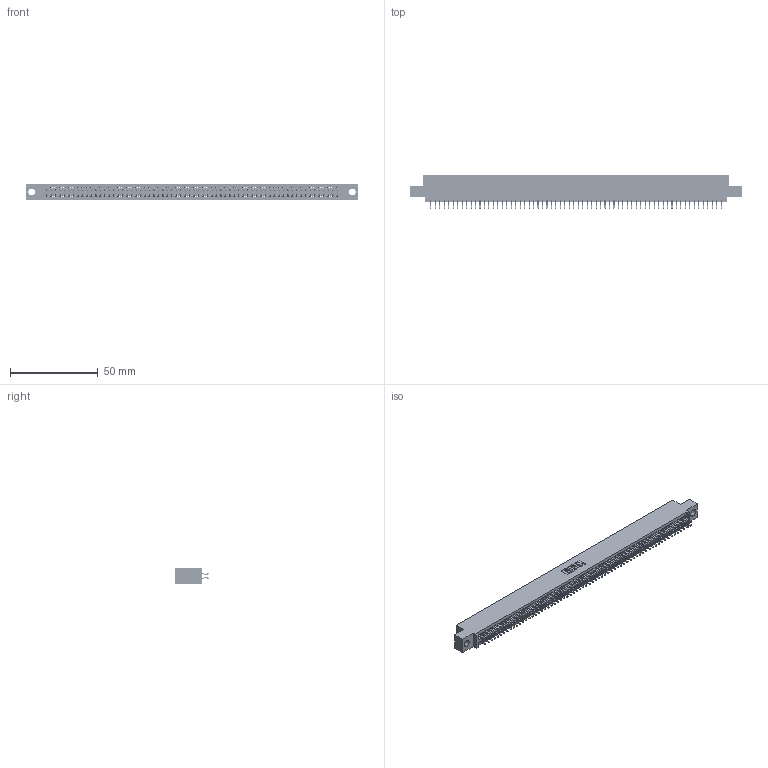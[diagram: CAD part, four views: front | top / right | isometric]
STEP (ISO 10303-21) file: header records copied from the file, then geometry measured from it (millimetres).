
FILE_DESCRIPTION (( 'STEP AP203' ), '1' );
FILE_NAME ('395-132-556-504.STEP', '2018-12-04T23:47:47', ( '' ), ( '' ), 'SwSTEP 2.0', 'SolidWorks 2016', '' );
FILE_SCHEMA (( 'CONFIG_CONTROL_DESIGN' ));
Length unit declared in the file: inch
Products named in the file (3): 395-132-556-504; 345-292-001_556 Tail; 345 Part_0.110 Offset - 0.156 Dia-TH
Assembly tree (133 placements, depth 2):
  395-132-556-504
    345 Part_0.110 Offset - 0.156 Dia-TH
    345-292-001_556 Tail  x132
Bounding box: 188.85 x 19.24 x 9.4 mm (x, y, z)
Volume: 18401.3 mm3; surface area: 27457.5 mm2
Topology: 133 solids, 133 shells, 7522 faces, 22397 edges, 14754 vertices
Faces by surface type: plane 4968, cylinder 2554
Entity records: 48909 total; most frequent: CARTESIAN_POINT 8192, ORIENTED_EDGE 8114, DIRECTION 7181, EDGE_CURVE 4057, LINE 3653, VECTOR 3653, VERTEX_POINT 2702, AXIS2_PLACEMENT_3D 1764
